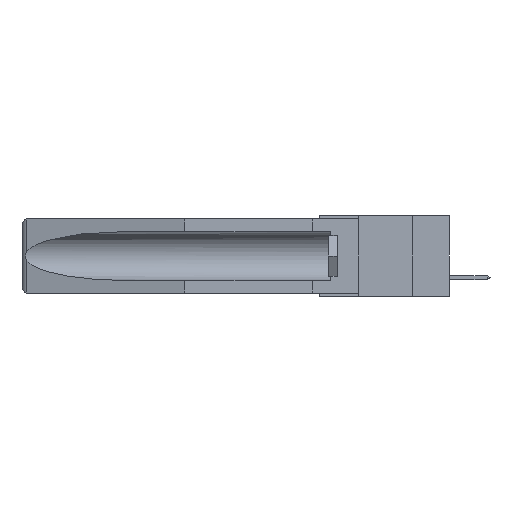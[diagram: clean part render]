
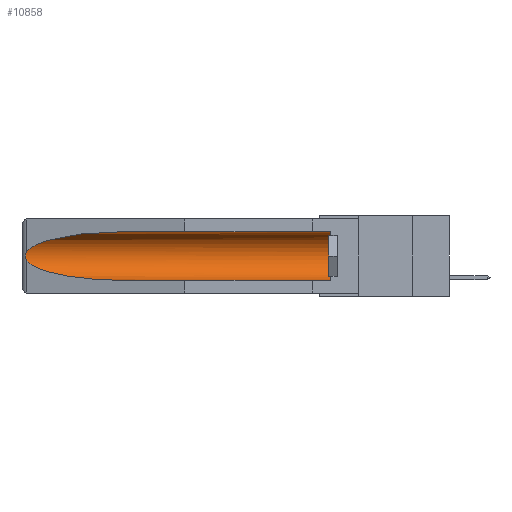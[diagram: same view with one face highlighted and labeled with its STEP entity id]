
A CAD part, left-side view. The second image highlights one B-rep face of the part: STEP entity #10858.
In plain terms, the highlighted cylindrical face has radius 2.857 mm (diameter 5.715 mm), a partial arc.
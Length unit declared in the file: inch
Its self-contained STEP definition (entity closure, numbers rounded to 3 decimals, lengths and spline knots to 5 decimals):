
#588 = CARTESIAN_POINT ( 'NONE',  ( 0.155, 1.07973, -0.284 ) ) ;
#1023 = CARTESIAN_POINT ( 'NONE',  ( 0.155, 1.07973, -0.284 ) ) ;
#1266 = CARTESIAN_POINT ( 'NONE',  ( 0.26537, 1.52718, -0.14972 ) ) ;
#1323 = ORIENTED_EDGE ( 'NONE', *, *, #6477, .T. ) ;
#1349 = ORIENTED_EDGE ( 'NONE', *, *, #14269, .T. ) ;
#1815 = CARTESIAN_POINT ( 'NONE',  ( 0.155, -0.30754, -0.284 ) ) ;
#2260 = CARTESIAN_POINT ( 'NONE',  ( 0.155, 0.126, -0.1715 ) ) ;
#2985 = CARTESIAN_POINT ( 'NONE',  ( 0.155, -0.30754, -0.059 ) ) ;
#3941 = VERTEX_POINT ( 'NONE', #12677 ) ;
#4739 = DIRECTION ( 'NONE',  ( 0., 0., 1. ) ) ;
#5021 = ORIENTED_EDGE ( 'NONE', *, *, #12536, .T. ) ;
#5484 = VERTEX_POINT ( 'NONE', #20479 ) ;
#5929 =( BOUNDED_CURVE ( )  B_SPLINE_CURVE ( 3, ( #8547, #13713, #25855, #31071 ),
 .UNSPECIFIED., .F., .F. ) 
 B_SPLINE_CURVE_WITH_KNOTS ( ( 4, 4 ),
 ( 4.71239, 6.08839 ),
 .UNSPECIFIED. ) 
 CURVE ( )  GEOMETRIC_REPRESENTATION_ITEM ( )  RATIONAL_B_SPLINE_CURVE ( ( 1., 0.848, 0.848, 1. ) ) 
 REPRESENTATION_ITEM ( '' )  );
#6477 = EDGE_CURVE ( 'NONE', #14701, #5484, #16954, .T. ) ;
#6480 = CARTESIAN_POINT ( 'NONE',  ( 0.26654, 1.53092, -0.15636 ) ) ;
#8232 = ORIENTED_EDGE ( 'NONE', *, *, #27828, .T. ) ;
#8547 = CARTESIAN_POINT ( 'NONE',  ( 0.155, 1.07973, -0.059 ) ) ;
#8691 = CYLINDRICAL_SURFACE ( 'NONE', #18909, 0.1125 ) ;
#8889 = CARTESIAN_POINT ( 'NONE',  ( 0.155, -0.30754, -0.1715 ) ) ;
#9083 = CARTESIAN_POINT ( 'NONE',  ( 0.2673, 1.53269, -0.17917 ) ) ;
#9298 = CARTESIAN_POINT ( 'NONE',  ( 0.155, 1.07973, -0.059 ) ) ;
#9926 = CARTESIAN_POINT ( 'NONE',  ( 0.155, 0.126, -0.284 ) ) ;
#10858 = ADVANCED_FACE ( 'NONE', ( #21865 ), #8691, .F. ) ;
#11235 = B_SPLINE_CURVE_WITH_KNOTS ( 'NONE', 3,
 ( #1266, #18791, #6480, #23567, #26283, #13930, #9083, #28561, #31722, #12092 ),
 .UNSPECIFIED., .F., .F.,
 ( 4, 2, 2, 2, 4 ),
 ( 0., 0.00029, 0.00058, 0.00087, 0.00117 ),
 .UNSPECIFIED. ) ;
#11253 = CARTESIAN_POINT ( 'NONE',  ( 0.26537, 1.52718, -0.19328 ) ) ;
#12092 = CARTESIAN_POINT ( 'NONE',  ( 0.26537, 1.52718, -0.19328 ) ) ;
#12536 = EDGE_CURVE ( 'NONE', #17471, #3941, #5929, .T. ) ;
#12677 = CARTESIAN_POINT ( 'NONE',  ( 0.26537, 1.52718, -0.14972 ) ) ;
#13713 = CARTESIAN_POINT ( 'NONE',  ( 0.21114, 1.30732, -0.059 ) ) ;
#13930 = CARTESIAN_POINT ( 'NONE',  ( 0.2675, 1.53308, -0.17534 ) ) ;
#14269 = EDGE_CURVE ( 'NONE', #3941, #23347, #11235, .T. ) ;
#14407 = DIRECTION ( 'NONE',  ( 0., 1., 0. ) ) ;
#14701 = VERTEX_POINT ( 'NONE', #9926 ) ;
#14717 = AXIS2_PLACEMENT_3D ( 'NONE', #2260, #19557, #4739 ) ;
#14992 = VECTOR ( 'NONE', #21591, 39.37008 ) ;
#15053 =( BOUNDED_CURVE ( )  B_SPLINE_CURVE ( 3, ( #11253, #23733, #25684, #1023 ),
 .UNSPECIFIED., .F., .F. ) 
 B_SPLINE_CURVE_WITH_KNOTS ( ( 4, 4 ),
 ( 0.1948, 1.5708 ),
 .UNSPECIFIED. ) 
 CURVE ( )  GEOMETRIC_REPRESENTATION_ITEM ( )  RATIONAL_B_SPLINE_CURVE ( ( 1., 0.848, 0.848, 1. ) ) 
 REPRESENTATION_ITEM ( '' )  );
#15181 = CARTESIAN_POINT ( 'NONE',  ( 0.26537, 1.52718, -0.19328 ) ) ;
#15294 = DIRECTION ( 'NONE',  ( 0., 1., 0. ) ) ;
#16325 = EDGE_LOOP ( 'NONE', ( #5021, #1349, #23744, #19837, #1323, #8232 ) ) ;
#16954 = CIRCLE ( 'NONE', #14717, 0.1125 ) ;
#17216 = VERTEX_POINT ( 'NONE', #588 ) ;
#17471 = VERTEX_POINT ( 'NONE', #9298 ) ;
#18791 = CARTESIAN_POINT ( 'NONE',  ( 0.26597, 1.52961, -0.15275 ) ) ;
#18909 = AXIS2_PLACEMENT_3D ( 'NONE', #8889, #14407, #26317 ) ;
#19557 = DIRECTION ( 'NONE',  ( 0., -1., 0. ) ) ;
#19837 = ORIENTED_EDGE ( 'NONE', *, *, #20179, .F. ) ;
#20179 = EDGE_CURVE ( 'NONE', #14701, #17216, #23894, .T. ) ;
#20479 = CARTESIAN_POINT ( 'NONE',  ( 0.155, 0.126, -0.059 ) ) ;
#21591 = DIRECTION ( 'NONE',  ( 0., 1., 0. ) ) ;
#21865 = FACE_OUTER_BOUND ( 'NONE', #16325, .T. ) ;
#22337 = LINE ( 'NONE', #2985, #29700 ) ;
#23347 = VERTEX_POINT ( 'NONE', #15181 ) ;
#23567 = CARTESIAN_POINT ( 'NONE',  ( 0.2673, 1.5327, -0.16383 ) ) ;
#23733 = CARTESIAN_POINT ( 'NONE',  ( 0.25451, 1.48313, -0.24835 ) ) ;
#23744 = ORIENTED_EDGE ( 'NONE', *, *, #25276, .T. ) ;
#23894 = LINE ( 'NONE', #1815, #14992 ) ;
#25276 = EDGE_CURVE ( 'NONE', #23347, #17216, #15053, .T. ) ;
#25684 = CARTESIAN_POINT ( 'NONE',  ( 0.21114, 1.30732, -0.284 ) ) ;
#25855 = CARTESIAN_POINT ( 'NONE',  ( 0.25451, 1.48313, -0.09465 ) ) ;
#26283 = CARTESIAN_POINT ( 'NONE',  ( 0.2675, 1.53308, -0.16763 ) ) ;
#26317 = DIRECTION ( 'NONE',  ( 0., 0., 1. ) ) ;
#27828 = EDGE_CURVE ( 'NONE', #5484, #17471, #22337, .T. ) ;
#28561 = CARTESIAN_POINT ( 'NONE',  ( 0.26655, 1.53094, -0.18657 ) ) ;
#29700 = VECTOR ( 'NONE', #15294, 39.37008 ) ;
#31071 = CARTESIAN_POINT ( 'NONE',  ( 0.26537, 1.52718, -0.14972 ) ) ;
#31722 = CARTESIAN_POINT ( 'NONE',  ( 0.26597, 1.5296, -0.19026 ) ) ;
